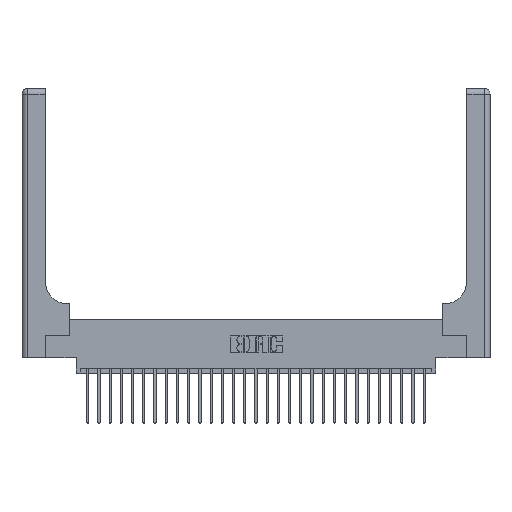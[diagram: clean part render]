
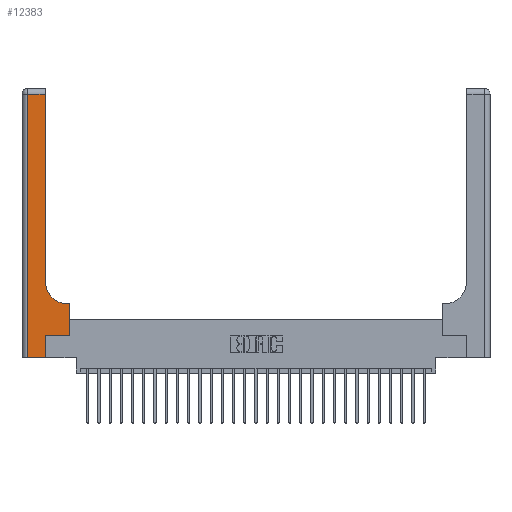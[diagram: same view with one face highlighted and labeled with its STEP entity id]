
A CAD part, top view. The second image highlights one B-rep face of the part: STEP entity #12383.
In plain terms, the highlighted planar face has unit normal (0, 0, 1).
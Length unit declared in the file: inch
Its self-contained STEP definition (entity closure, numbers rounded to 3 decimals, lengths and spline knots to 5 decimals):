
#639 = DIRECTION ( 'NONE',  ( -1., 0., 0. ) ) ;
#708 = EDGE_CURVE ( 'NONE', #1648, #7507, #23449, .T. ) ;
#962 = VERTEX_POINT ( 'NONE', #24875 ) ;
#1025 = DIRECTION ( 'NONE',  ( 0., -1., 0. ) ) ;
#1360 = VECTOR ( 'NONE', #19448, 39.37008 ) ;
#1648 = VERTEX_POINT ( 'NONE', #2077 ) ;
#1992 = DIRECTION ( 'NONE',  ( 0., 0., -1. ) ) ;
#2077 = CARTESIAN_POINT ( 'NONE',  ( 0.26, 2.94, 0.37 ) ) ;
#2696 = CARTESIAN_POINT ( 'NONE',  ( 0., 3., 0.37 ) ) ;
#2806 = AXIS2_PLACEMENT_3D ( 'NONE', #14530, #1992, #16615 ) ;
#2970 = FACE_OUTER_BOUND ( 'NONE', #12162, .T. ) ;
#3247 = ORIENTED_EDGE ( 'NONE', *, *, #17938, .T. ) ;
#3907 = DIRECTION ( 'NONE',  ( 1., 0., 0. ) ) ;
#4409 = EDGE_CURVE ( 'NONE', #24643, #1648, #5691, .T. ) ;
#5084 = DIRECTION ( 'NONE',  ( 1., 0., 0. ) ) ;
#5185 = ORIENTED_EDGE ( 'NONE', *, *, #23697, .T. ) ;
#5547 = CIRCLE ( 'NONE', #2806, 0.25 ) ;
#5691 = LINE ( 'NONE', #7953, #16855 ) ;
#6832 = ORIENTED_EDGE ( 'NONE', *, *, #4409, .T. ) ;
#7080 = LINE ( 'NONE', #11465, #17584 ) ;
#7305 = CARTESIAN_POINT ( 'NONE',  ( 0., 2.94, 0.37 ) ) ;
#7507 = VERTEX_POINT ( 'NONE', #19803 ) ;
#7577 = LINE ( 'NONE', #8974, #1360 ) ;
#7872 = VERTEX_POINT ( 'NONE', #18801 ) ;
#7953 = CARTESIAN_POINT ( 'NONE',  ( 0.26, 3., 0.37 ) ) ;
#8974 = CARTESIAN_POINT ( 'NONE',  ( 0.528, 0.25, 0.37 ) ) ;
#9288 = VECTOR ( 'NONE', #13709, 39.37008 ) ;
#9806 = CARTESIAN_POINT ( 'NONE',  ( 0.26, 0.85, 0.37 ) ) ;
#10284 = VECTOR ( 'NONE', #3907, 39.37008 ) ;
#10680 = AXIS2_PLACEMENT_3D ( 'NONE', #2696, #13212, #639 ) ;
#10767 = VERTEX_POINT ( 'NONE', #19596 ) ;
#10816 = LINE ( 'NONE', #13439, #21302 ) ;
#11460 = VECTOR ( 'NONE', #16897, 39.37008 ) ;
#11465 = CARTESIAN_POINT ( 'NONE',  ( 0.06, 3., 0.37 ) ) ;
#12162 = EDGE_LOOP ( 'NONE', ( #6832, #13067, #18644, #19308, #3247, #15034, #15684, #26762, #5185 ) ) ;
#12318 = VECTOR ( 'NONE', #21981, 39.37008 ) ;
#12383 = ADVANCED_FACE ( 'NONE', ( #2970 ), #25693, .F. ) ;
#13067 = ORIENTED_EDGE ( 'NONE', *, *, #708, .T. ) ;
#13212 = DIRECTION ( 'NONE',  ( 0., 0., -1. ) ) ;
#13214 = EDGE_CURVE ( 'NONE', #7872, #22652, #10816, .T. ) ;
#13244 = CARTESIAN_POINT ( 'NONE',  ( 0.528, 0.25, 0.37 ) ) ;
#13439 = CARTESIAN_POINT ( 'NONE',  ( 0., 0., 0.37 ) ) ;
#13709 = DIRECTION ( 'NONE',  ( 0., 1., 0. ) ) ;
#14530 = CARTESIAN_POINT ( 'NONE',  ( 0.51, 0.85, 0.37 ) ) ;
#14785 = CARTESIAN_POINT ( 'NONE',  ( 0.265, 0., 0.37 ) ) ;
#15034 = ORIENTED_EDGE ( 'NONE', *, *, #18156, .T. ) ;
#15684 = ORIENTED_EDGE ( 'NONE', *, *, #22678, .T. ) ;
#16441 = CARTESIAN_POINT ( 'NONE',  ( 0.265, 0.25, 0.37 ) ) ;
#16542 = VERTEX_POINT ( 'NONE', #13244 ) ;
#16615 = DIRECTION ( 'NONE',  ( 1., 0., 0. ) ) ;
#16855 = VECTOR ( 'NONE', #22631, 39.37008 ) ;
#16897 = DIRECTION ( 'NONE',  ( -1., 0., 0. ) ) ;
#17040 = LINE ( 'NONE', #21044, #11460 ) ;
#17584 = VECTOR ( 'NONE', #1025, 39.37008 ) ;
#17938 = EDGE_CURVE ( 'NONE', #22652, #10767, #19791, .T. ) ;
#18156 = EDGE_CURVE ( 'NONE', #10767, #16542, #26259, .T. ) ;
#18644 = ORIENTED_EDGE ( 'NONE', *, *, #26451, .T. ) ;
#18801 = CARTESIAN_POINT ( 'NONE',  ( 0.06, 0., 0.37 ) ) ;
#19308 = ORIENTED_EDGE ( 'NONE', *, *, #13214, .T. ) ;
#19448 = DIRECTION ( 'NONE',  ( 0., 1., 0. ) ) ;
#19596 = CARTESIAN_POINT ( 'NONE',  ( 0.265, 0.25, 0.37 ) ) ;
#19791 = LINE ( 'NONE', #26191, #9288 ) ;
#19803 = CARTESIAN_POINT ( 'NONE',  ( 0.06, 2.94, 0.37 ) ) ;
#20586 = EDGE_CURVE ( 'NONE', #21230, #962, #17040, .T. ) ;
#21044 = CARTESIAN_POINT ( 'NONE',  ( 0.26, 0.6, 0.37 ) ) ;
#21230 = VERTEX_POINT ( 'NONE', #25171 ) ;
#21302 = VECTOR ( 'NONE', #5084, 39.37008 ) ;
#21981 = DIRECTION ( 'NONE',  ( -1., 0., 0. ) ) ;
#22631 = DIRECTION ( 'NONE',  ( 0., 1., 0. ) ) ;
#22652 = VERTEX_POINT ( 'NONE', #14785 ) ;
#22678 = EDGE_CURVE ( 'NONE', #16542, #21230, #7577, .T. ) ;
#23449 = LINE ( 'NONE', #7305, #12318 ) ;
#23697 = EDGE_CURVE ( 'NONE', #962, #24643, #5547, .T. ) ;
#24643 = VERTEX_POINT ( 'NONE', #9806 ) ;
#24875 = CARTESIAN_POINT ( 'NONE',  ( 0.51, 0.6, 0.37 ) ) ;
#25171 = CARTESIAN_POINT ( 'NONE',  ( 0.528, 0.6, 0.37 ) ) ;
#25693 = PLANE ( 'NONE',  #10680 ) ;
#26191 = CARTESIAN_POINT ( 'NONE',  ( 0.265, 0., 0.37 ) ) ;
#26259 = LINE ( 'NONE', #16441, #10284 ) ;
#26451 = EDGE_CURVE ( 'NONE', #7507, #7872, #7080, .T. ) ;
#26762 = ORIENTED_EDGE ( 'NONE', *, *, #20586, .T. ) ;
